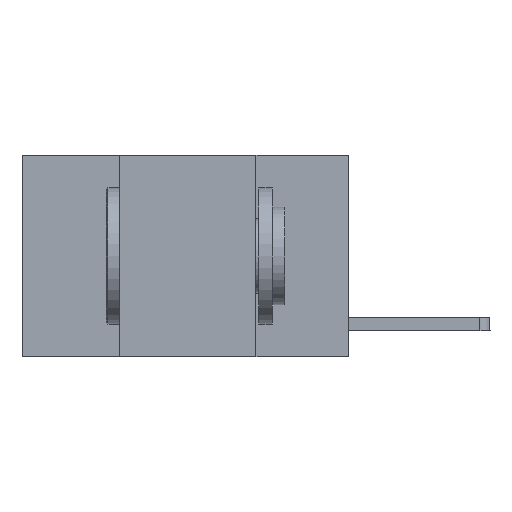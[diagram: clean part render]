
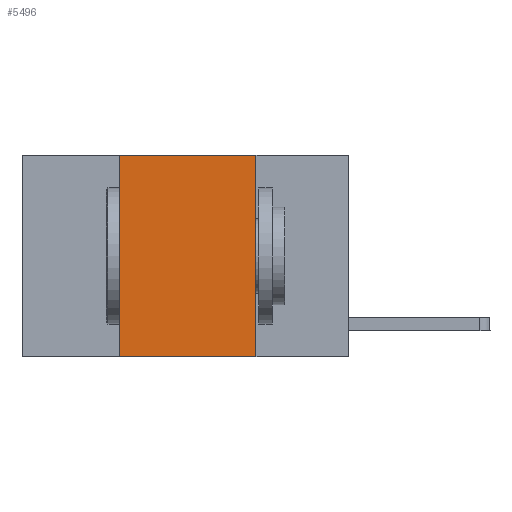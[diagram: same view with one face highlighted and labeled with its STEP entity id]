
A CAD part, left-side view. The second image highlights one B-rep face of the part: STEP entity #5496.
In plain terms, the highlighted planar face has unit normal (-1, 0, 0).
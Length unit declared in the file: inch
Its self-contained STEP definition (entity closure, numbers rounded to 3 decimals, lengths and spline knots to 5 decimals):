
#80 = ORIENTED_EDGE ( 'NONE', *, *, #11404, .T. ) ;
#687 = VERTEX_POINT ( 'NONE', #4995 ) ;
#691 = CARTESIAN_POINT ( 'NONE',  ( 0., 0.6, 0. ) ) ;
#698 = EDGE_CURVE ( 'NONE', #6396, #2464, #10628, .T. ) ;
#870 = AXIS2_PLACEMENT_3D ( 'NONE', #691, #2794, #11991 ) ;
#1623 = PLANE ( 'NONE',  #870 ) ;
#1640 = VERTEX_POINT ( 'NONE', #7997 ) ;
#2464 = VERTEX_POINT ( 'NONE', #11762 ) ;
#2794 = DIRECTION ( 'NONE',  ( 1., 0., 0. ) ) ;
#3340 = CARTESIAN_POINT ( 'NONE',  ( 0., 0.17, 0. ) ) ;
#4622 = CARTESIAN_POINT ( 'NONE',  ( 0., 0.17, 0. ) ) ;
#4995 = CARTESIAN_POINT ( 'NONE',  ( 0., 0.42, -0.37 ) ) ;
#5186 = VECTOR ( 'NONE', #10688, 39.37008 ) ;
#5192 = DIRECTION ( 'NONE',  ( 0., -1., 0. ) ) ;
#5317 = EDGE_CURVE ( 'NONE', #687, #1640, #8097, .T. ) ;
#5496 = ADVANCED_FACE ( 'NONE', ( #11187 ), #1623, .F. ) ;
#6396 = VERTEX_POINT ( 'NONE', #4622 ) ;
#6400 = CARTESIAN_POINT ( 'NONE',  ( 0., 0.6, -0.37 ) ) ;
#6470 = EDGE_LOOP ( 'NONE', ( #9909, #11572, #8953, #80 ) ) ;
#6589 = VECTOR ( 'NONE', #8238, 39.37008 ) ;
#7997 = CARTESIAN_POINT ( 'NONE',  ( 0., 0.42, 0. ) ) ;
#8097 = LINE ( 'NONE', #10626, #11051 ) ;
#8238 = DIRECTION ( 'NONE',  ( 0., -1., 0. ) ) ;
#8952 = VECTOR ( 'NONE', #5192, 39.37008 ) ;
#8953 = ORIENTED_EDGE ( 'NONE', *, *, #5317, .F. ) ;
#9909 = ORIENTED_EDGE ( 'NONE', *, *, #698, .F. ) ;
#9961 = CARTESIAN_POINT ( 'NONE',  ( 0., 0.6, 0. ) ) ;
#10626 = CARTESIAN_POINT ( 'NONE',  ( 0., 0.42, 0. ) ) ;
#10628 = LINE ( 'NONE', #3340, #5186 ) ;
#10688 = DIRECTION ( 'NONE',  ( 0., 0., -1. ) ) ;
#10928 = LINE ( 'NONE', #6400, #6589 ) ;
#11051 = VECTOR ( 'NONE', #11486, 39.37008 ) ;
#11187 = FACE_OUTER_BOUND ( 'NONE', #6470, .T. ) ;
#11213 = EDGE_CURVE ( 'NONE', #1640, #6396, #11631, .T. ) ;
#11404 = EDGE_CURVE ( 'NONE', #687, #2464, #10928, .T. ) ;
#11486 = DIRECTION ( 'NONE',  ( 0., 0., 1. ) ) ;
#11572 = ORIENTED_EDGE ( 'NONE', *, *, #11213, .F. ) ;
#11631 = LINE ( 'NONE', #9961, #8952 ) ;
#11762 = CARTESIAN_POINT ( 'NONE',  ( 0., 0.17, -0.37 ) ) ;
#11991 = DIRECTION ( 'NONE',  ( 0., 0., -1. ) ) ;
